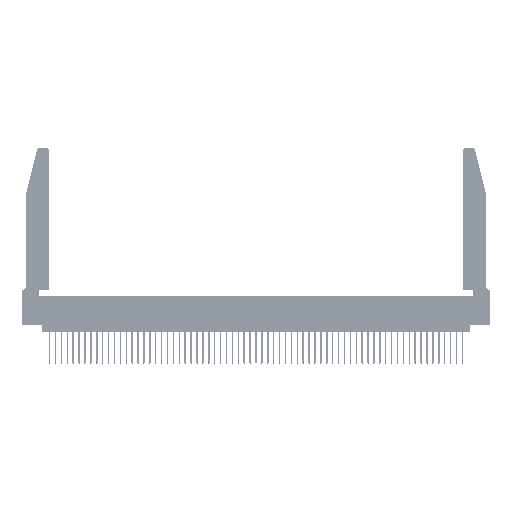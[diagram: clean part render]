
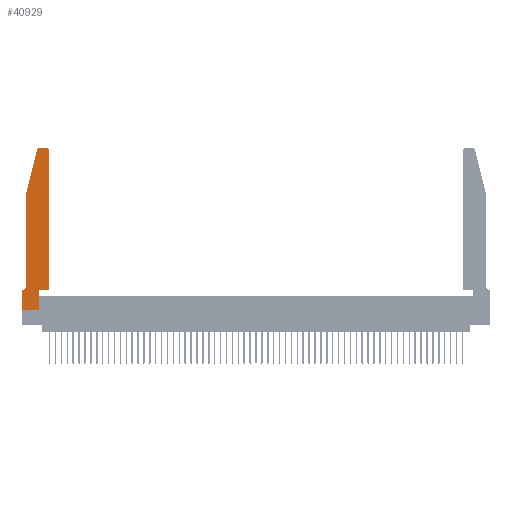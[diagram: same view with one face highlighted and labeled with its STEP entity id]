
A CAD part, top view. The second image highlights one B-rep face of the part: STEP entity #40929.
In plain terms, the highlighted planar face has unit normal (0, 0, 1).
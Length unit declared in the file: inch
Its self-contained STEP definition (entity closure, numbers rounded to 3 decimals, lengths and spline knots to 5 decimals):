
#78 = CARTESIAN_POINT ( 'NONE',  ( 0.25487, 2.72718, 0.37 ) ) ;
#184 = EDGE_CURVE ( 'NONE', #49687, #12855, #8437, .T. ) ;
#529 = CARTESIAN_POINT ( 'NONE',  ( 0.4205, 2.72, 0.37 ) ) ;
#987 = DIRECTION ( 'NONE',  ( -0.239, -0.971, 0. ) ) ;
#1336 = VECTOR ( 'NONE', #4804, 39.37008 ) ;
#1601 = CARTESIAN_POINT ( 'NONE',  ( 0.2865, 0., 0.37 ) ) ;
#1739 = CARTESIAN_POINT ( 'NONE',  ( 0., 0.35, 0.37 ) ) ;
#1981 = ORIENTED_EDGE ( 'NONE', *, *, #23024, .T. ) ;
#2833 = LINE ( 'NONE', #52836, #49481 ) ;
#3877 = AXIS2_PLACEMENT_3D ( 'NONE', #529, #31361, #4992 ) ;
#4804 = DIRECTION ( 'NONE',  ( -1., 0., 0. ) ) ;
#4889 = LINE ( 'NONE', #27895, #26934 ) ;
#4992 = DIRECTION ( 'NONE',  ( 1., 0., 0. ) ) ;
#5318 = EDGE_CURVE ( 'NONE', #47554, #11802, #15834, .T. ) ;
#5374 = VECTOR ( 'NONE', #47920, 39.37008 ) ;
#5950 = DIRECTION ( 'NONE',  ( 0., -1., 0. ) ) ;
#6852 = VERTEX_POINT ( 'NONE', #50200 ) ;
#6992 = EDGE_CURVE ( 'NONE', #49159, #29206, #32853, .T. ) ;
#7456 = DIRECTION ( 'NONE',  ( 0., 0., 1. ) ) ;
#7786 = ORIENTED_EDGE ( 'NONE', *, *, #184, .T. ) ;
#7802 = ORIENTED_EDGE ( 'NONE', *, *, #6992, .T. ) ;
#8437 = LINE ( 'NONE', #38371, #20129 ) ;
#8481 = AXIS2_PLACEMENT_3D ( 'NONE', #18797, #49399, #23213 ) ;
#8661 = LINE ( 'NONE', #16902, #18972 ) ;
#9376 = AXIS2_PLACEMENT_3D ( 'NONE', #33825, #7456, #38200 ) ;
#10073 = CIRCLE ( 'NONE', #8481, 0.07 ) ;
#10634 = PLANE ( 'NONE',  #31647 ) ;
#11033 = EDGE_CURVE ( 'NONE', #34270, #49687, #17063, .T. ) ;
#11802 = VERTEX_POINT ( 'NONE', #44023 ) ;
#11956 = CARTESIAN_POINT ( 'NONE',  ( 0., 0., 0.37 ) ) ;
#11971 = ORIENTED_EDGE ( 'NONE', *, *, #11033, .T. ) ;
#12065 = DIRECTION ( 'NONE',  ( 0., 1., 0. ) ) ;
#12318 = FACE_OUTER_BOUND ( 'NONE', #39722, .T. ) ;
#12691 = DIRECTION ( 'NONE',  ( 1., 0., 0. ) ) ;
#12855 = VERTEX_POINT ( 'NONE', #48335 ) ;
#14169 = CARTESIAN_POINT ( 'NONE',  ( 0.4205, 2.75, 0.37 ) ) ;
#14480 = VERTEX_POINT ( 'NONE', #41531 ) ;
#15038 = DIRECTION ( 'NONE',  ( 0., 0., 1. ) ) ;
#15577 = CARTESIAN_POINT ( 'NONE',  ( 0., 0.35, 0.37 ) ) ;
#15834 = LINE ( 'NONE', #39973, #1336 ) ;
#16902 = CARTESIAN_POINT ( 'NONE',  ( 0.4505, 0.35, 0.37 ) ) ;
#17063 = LINE ( 'NONE', #52249, #5374 ) ;
#17138 = VECTOR ( 'NONE', #987, 39.37008 ) ;
#18797 = CARTESIAN_POINT ( 'NONE',  ( 0.0055, 0.42, 0.37 ) ) ;
#18972 = VECTOR ( 'NONE', #12691, 39.37008 ) ;
#20129 = VECTOR ( 'NONE', #12065, 39.37008 ) ;
#20567 = CARTESIAN_POINT ( 'NONE',  ( 0.0755, 0.35, 0.37 ) ) ;
#22316 = DIRECTION ( 'NONE',  ( 0., -1., 0. ) ) ;
#22902 = ORIENTED_EDGE ( 'NONE', *, *, #23388, .T. ) ;
#23024 = EDGE_CURVE ( 'NONE', #49070, #6852, #2833, .T. ) ;
#23136 = CARTESIAN_POINT ( 'NONE',  ( 0.4505, 2.72, 0.37 ) ) ;
#23213 = DIRECTION ( 'NONE',  ( -1., 0., 0. ) ) ;
#23388 = EDGE_CURVE ( 'NONE', #11802, #26350, #28951, .T. ) ;
#26350 = VERTEX_POINT ( 'NONE', #78 ) ;
#26934 = VECTOR ( 'NONE', #5950, 39.37008 ) ;
#27537 = EDGE_CURVE ( 'NONE', #12855, #14480, #8661, .T. ) ;
#27895 = CARTESIAN_POINT ( 'NONE',  ( 0., 0., 0.37 ) ) ;
#28040 = CARTESIAN_POINT ( 'NONE',  ( 0.0755, 2., 0.37 ) ) ;
#28951 = CIRCLE ( 'NONE', #9376, 0.03 ) ;
#29206 = VERTEX_POINT ( 'NONE', #15577 ) ;
#29332 = EDGE_CURVE ( 'NONE', #14480, #33955, #53601, .T. ) ;
#30090 = EDGE_CURVE ( 'NONE', #29206, #34270, #4889, .T. ) ;
#31233 = EDGE_CURVE ( 'NONE', #26350, #49070, #33013, .T. ) ;
#31361 = DIRECTION ( 'NONE',  ( 0., 0., 1. ) ) ;
#31647 = AXIS2_PLACEMENT_3D ( 'NONE', #1739, #15038, #45677 ) ;
#32853 = LINE ( 'NONE', #20567, #53239 ) ;
#33013 = LINE ( 'NONE', #36249, #17138 ) ;
#33825 = CARTESIAN_POINT ( 'NONE',  ( 0.284, 2.72, 0.37 ) ) ;
#33866 = CARTESIAN_POINT ( 'NONE',  ( 0.4505, 0.35, 0.37 ) ) ;
#33955 = VERTEX_POINT ( 'NONE', #23136 ) ;
#34270 = VERTEX_POINT ( 'NONE', #11956 ) ;
#35655 = ORIENTED_EDGE ( 'NONE', *, *, #27537, .T. ) ;
#36249 = CARTESIAN_POINT ( 'NONE',  ( 0.0755, 2., 0.37 ) ) ;
#38200 = DIRECTION ( 'NONE',  ( 1., 0., 0. ) ) ;
#38371 = CARTESIAN_POINT ( 'NONE',  ( 0.2865, 0.35, 0.37 ) ) ;
#38880 = ORIENTED_EDGE ( 'NONE', *, *, #50737, .T. ) ;
#39722 = EDGE_LOOP ( 'NONE', ( #44192, #22902, #49583, #1981, #47553, #7802, #55777, #11971, #7786, #35655, #41384, #38880 ) ) ;
#39973 = CARTESIAN_POINT ( 'NONE',  ( 0.2605, 2.75, 0.37 ) ) ;
#40929 = ADVANCED_FACE ( 'NONE', ( #12318 ), #10634, .T. ) ;
#41384 = ORIENTED_EDGE ( 'NONE', *, *, #29332, .T. ) ;
#41531 = CARTESIAN_POINT ( 'NONE',  ( 0.4505, 0.35, 0.37 ) ) ;
#42599 = EDGE_CURVE ( 'NONE', #6852, #49159, #10073, .T. ) ;
#44023 = CARTESIAN_POINT ( 'NONE',  ( 0.284, 2.75, 0.37 ) ) ;
#44192 = ORIENTED_EDGE ( 'NONE', *, *, #5318, .T. ) ;
#45677 = DIRECTION ( 'NONE',  ( 1., 0., 0. ) ) ;
#46963 = DIRECTION ( 'NONE',  ( 0., 1., 0. ) ) ;
#47553 = ORIENTED_EDGE ( 'NONE', *, *, #42599, .T. ) ;
#47554 = VERTEX_POINT ( 'NONE', #14169 ) ;
#47920 = DIRECTION ( 'NONE',  ( 1., 0., 0. ) ) ;
#48335 = CARTESIAN_POINT ( 'NONE',  ( 0.2865, 0.35, 0.37 ) ) ;
#49070 = VERTEX_POINT ( 'NONE', #28040 ) ;
#49159 = VERTEX_POINT ( 'NONE', #54706 ) ;
#49399 = DIRECTION ( 'NONE',  ( 0., 0., -1. ) ) ;
#49481 = VECTOR ( 'NONE', #22316, 39.37008 ) ;
#49583 = ORIENTED_EDGE ( 'NONE', *, *, #31233, .T. ) ;
#49687 = VERTEX_POINT ( 'NONE', #1601 ) ;
#50200 = CARTESIAN_POINT ( 'NONE',  ( 0.0755, 0.42, 0.37 ) ) ;
#50737 = EDGE_CURVE ( 'NONE', #33955, #47554, #52762, .T. ) ;
#52222 = VECTOR ( 'NONE', #46963, 39.37008 ) ;
#52249 = CARTESIAN_POINT ( 'NONE',  ( 0., 0., 0.37 ) ) ;
#52762 = CIRCLE ( 'NONE', #3877, 0.03 ) ;
#52836 = CARTESIAN_POINT ( 'NONE',  ( 0.0755, 2., 0.37 ) ) ;
#53239 = VECTOR ( 'NONE', #55507, 39.37008 ) ;
#53601 = LINE ( 'NONE', #33866, #52222 ) ;
#54706 = CARTESIAN_POINT ( 'NONE',  ( 0.0055, 0.35, 0.37 ) ) ;
#55507 = DIRECTION ( 'NONE',  ( -1., 0., 0. ) ) ;
#55777 = ORIENTED_EDGE ( 'NONE', *, *, #30090, .T. ) ;
